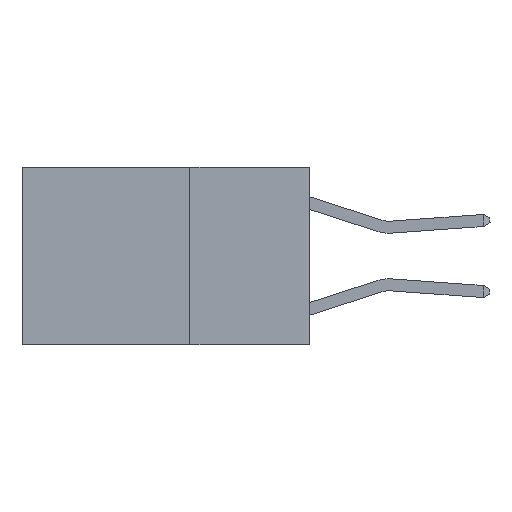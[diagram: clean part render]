
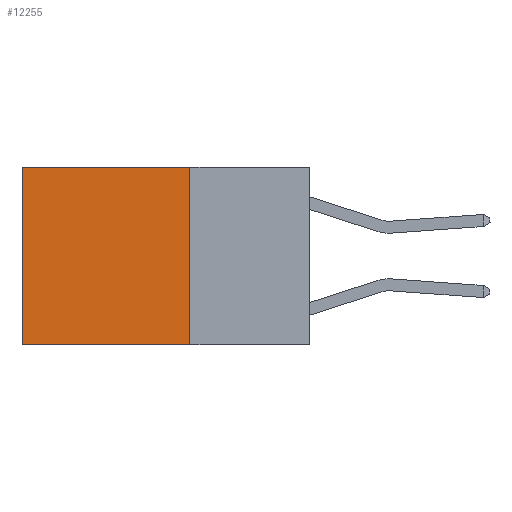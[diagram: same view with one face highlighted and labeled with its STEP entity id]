
A CAD part, left-side view. The second image highlights one B-rep face of the part: STEP entity #12255.
In plain terms, the highlighted planar face has unit normal (-1, 0, 0).
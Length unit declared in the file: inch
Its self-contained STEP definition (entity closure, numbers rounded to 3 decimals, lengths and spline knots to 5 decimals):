
#79 = VERTEX_POINT ( 'NONE', #18254 ) ;
#761 = CARTESIAN_POINT ( 'NONE',  ( 0.2625, 0.25, 0. ) ) ;
#868 = LINE ( 'NONE', #11282, #17274 ) ;
#2100 = DIRECTION ( 'NONE',  ( 0., 0., -1. ) ) ;
#2107 = DIRECTION ( 'NONE',  ( 0., 1., 0. ) ) ;
#3103 = ORIENTED_EDGE ( 'NONE', *, *, #14703, .T. ) ;
#3517 = FACE_OUTER_BOUND ( 'NONE', #14926, .T. ) ;
#3582 = CARTESIAN_POINT ( 'NONE',  ( 0.2625, 0.25, 0. ) ) ;
#3719 = CARTESIAN_POINT ( 'NONE',  ( 0.2625, 0.25, 0. ) ) ;
#3926 = PLANE ( 'NONE',  #14888 ) ;
#5776 = VECTOR ( 'NONE', #2107, 39.37008 ) ;
#6033 = CARTESIAN_POINT ( 'NONE',  ( 0.2625, 0.25, -0.37 ) ) ;
#7191 = CARTESIAN_POINT ( 'NONE',  ( 0.2625, 0.25, -0.37 ) ) ;
#8540 = DIRECTION ( 'NONE',  ( 0., 0., -1. ) ) ;
#8883 = LINE ( 'NONE', #3582, #5776 ) ;
#9047 = LINE ( 'NONE', #7191, #12678 ) ;
#9854 = VERTEX_POINT ( 'NONE', #19800 ) ;
#11282 = CARTESIAN_POINT ( 'NONE',  ( 0.2625, 0.6, 0. ) ) ;
#11363 = DIRECTION ( 'NONE',  ( 0., 0., -1. ) ) ;
#11677 = EDGE_CURVE ( 'NONE', #17707, #79, #9047, .T. ) ;
#12113 = LINE ( 'NONE', #3719, #16223 ) ;
#12255 = ADVANCED_FACE ( 'NONE', ( #3517 ), #3926, .F. ) ;
#12678 = VECTOR ( 'NONE', #17954, 39.37008 ) ;
#12906 = VERTEX_POINT ( 'NONE', #17763 ) ;
#13170 = ORIENTED_EDGE ( 'NONE', *, *, #16778, .T. ) ;
#14302 = ORIENTED_EDGE ( 'NONE', *, *, #18608, .F. ) ;
#14703 = EDGE_CURVE ( 'NONE', #9854, #12906, #8883, .T. ) ;
#14888 = AXIS2_PLACEMENT_3D ( 'NONE', #761, #17788, #8540 ) ;
#14926 = EDGE_LOOP ( 'NONE', ( #13170, #16100, #14302, #3103 ) ) ;
#16100 = ORIENTED_EDGE ( 'NONE', *, *, #11677, .F. ) ;
#16223 = VECTOR ( 'NONE', #11363, 39.37008 ) ;
#16778 = EDGE_CURVE ( 'NONE', #12906, #79, #868, .T. ) ;
#17274 = VECTOR ( 'NONE', #2100, 39.37008 ) ;
#17707 = VERTEX_POINT ( 'NONE', #6033 ) ;
#17763 = CARTESIAN_POINT ( 'NONE',  ( 0.2625, 0.6, 0. ) ) ;
#17788 = DIRECTION ( 'NONE',  ( 1., 0., 0. ) ) ;
#17954 = DIRECTION ( 'NONE',  ( 0., 1., 0. ) ) ;
#18254 = CARTESIAN_POINT ( 'NONE',  ( 0.2625, 0.6, -0.37 ) ) ;
#18608 = EDGE_CURVE ( 'NONE', #9854, #17707, #12113, .T. ) ;
#19800 = CARTESIAN_POINT ( 'NONE',  ( 0.2625, 0.25, 0. ) ) ;
